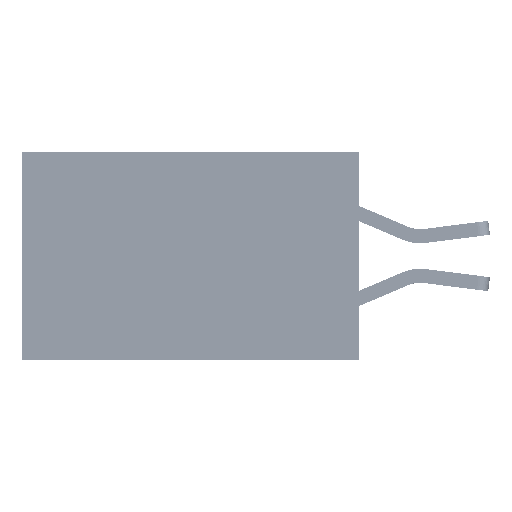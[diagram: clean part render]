
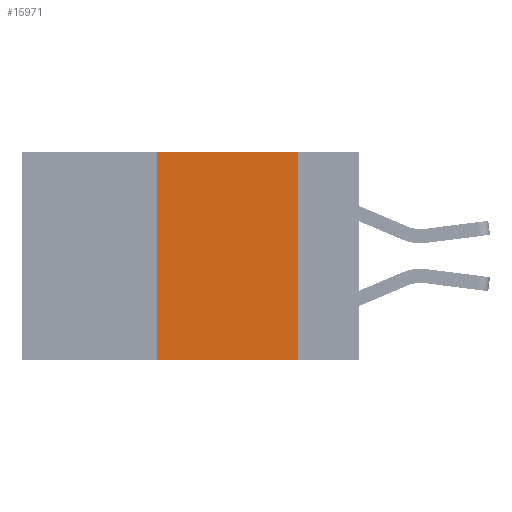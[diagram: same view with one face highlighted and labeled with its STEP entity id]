
A CAD part, left-side view. The second image highlights one B-rep face of the part: STEP entity #15971.
In plain terms, the highlighted planar face has unit normal (-1, 0, 0).
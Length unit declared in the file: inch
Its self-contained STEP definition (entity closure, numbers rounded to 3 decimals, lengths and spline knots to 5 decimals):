
#1208 = EDGE_CURVE ( 'NONE', #13434, #7125, #4109, .T. ) ;
#2003 = CARTESIAN_POINT ( 'NONE',  ( 0., 0.11, 0. ) ) ;
#2212 = PLANE ( 'NONE',  #14705 ) ;
#2473 = DIRECTION ( 'NONE',  ( 0., -1., 0. ) ) ;
#2726 = EDGE_LOOP ( 'NONE', ( #37968, #37117, #18384, #10558 ) ) ;
#4109 = LINE ( 'NONE', #22103, #29711 ) ;
#7125 = VERTEX_POINT ( 'NONE', #2003 ) ;
#8053 = EDGE_CURVE ( 'NONE', #7125, #25344, #19898, .T. ) ;
#8804 = CARTESIAN_POINT ( 'NONE',  ( 0., 0.6, -0.37 ) ) ;
#8978 = CARTESIAN_POINT ( 'NONE',  ( 0., 0.36, -0.37 ) ) ;
#10558 = ORIENTED_EDGE ( 'NONE', *, *, #37193, .T. ) ;
#10579 = DIRECTION ( 'NONE',  ( 0., 0., 1. ) ) ;
#11882 = FACE_OUTER_BOUND ( 'NONE', #2726, .T. ) ;
#13351 = CARTESIAN_POINT ( 'NONE',  ( 0., 0.36, 0. ) ) ;
#13434 = VERTEX_POINT ( 'NONE', #15030 ) ;
#14675 = CARTESIAN_POINT ( 'NONE',  ( 0., 0.6, 0. ) ) ;
#14705 = AXIS2_PLACEMENT_3D ( 'NONE', #14675, #23579, #26749 ) ;
#15030 = CARTESIAN_POINT ( 'NONE',  ( 0., 0.36, 0. ) ) ;
#15971 = ADVANCED_FACE ( 'NONE', ( #11882 ), #2212, .F. ) ;
#16920 = VERTEX_POINT ( 'NONE', #8978 ) ;
#18214 = CARTESIAN_POINT ( 'NONE',  ( 0., 0.11, -0.37 ) ) ;
#18384 = ORIENTED_EDGE ( 'NONE', *, *, #30261, .F. ) ;
#19898 = LINE ( 'NONE', #32009, #34539 ) ;
#22032 = VECTOR ( 'NONE', #10579, 39.37008 ) ;
#22103 = CARTESIAN_POINT ( 'NONE',  ( 0., 0.6, 0. ) ) ;
#23579 = DIRECTION ( 'NONE',  ( 1., 0., 0. ) ) ;
#25344 = VERTEX_POINT ( 'NONE', #18214 ) ;
#26016 = LINE ( 'NONE', #13351, #22032 ) ;
#26749 = DIRECTION ( 'NONE',  ( 0., 0., -1. ) ) ;
#29241 = DIRECTION ( 'NONE',  ( 0., 0., -1. ) ) ;
#29422 = LINE ( 'NONE', #8804, #31838 ) ;
#29711 = VECTOR ( 'NONE', #34197, 39.37008 ) ;
#30261 = EDGE_CURVE ( 'NONE', #16920, #13434, #26016, .T. ) ;
#31838 = VECTOR ( 'NONE', #2473, 39.37008 ) ;
#32009 = CARTESIAN_POINT ( 'NONE',  ( 0., 0.11, 0. ) ) ;
#34197 = DIRECTION ( 'NONE',  ( 0., -1., 0. ) ) ;
#34539 = VECTOR ( 'NONE', #29241, 39.37008 ) ;
#37117 = ORIENTED_EDGE ( 'NONE', *, *, #1208, .F. ) ;
#37193 = EDGE_CURVE ( 'NONE', #16920, #25344, #29422, .T. ) ;
#37968 = ORIENTED_EDGE ( 'NONE', *, *, #8053, .F. ) ;
